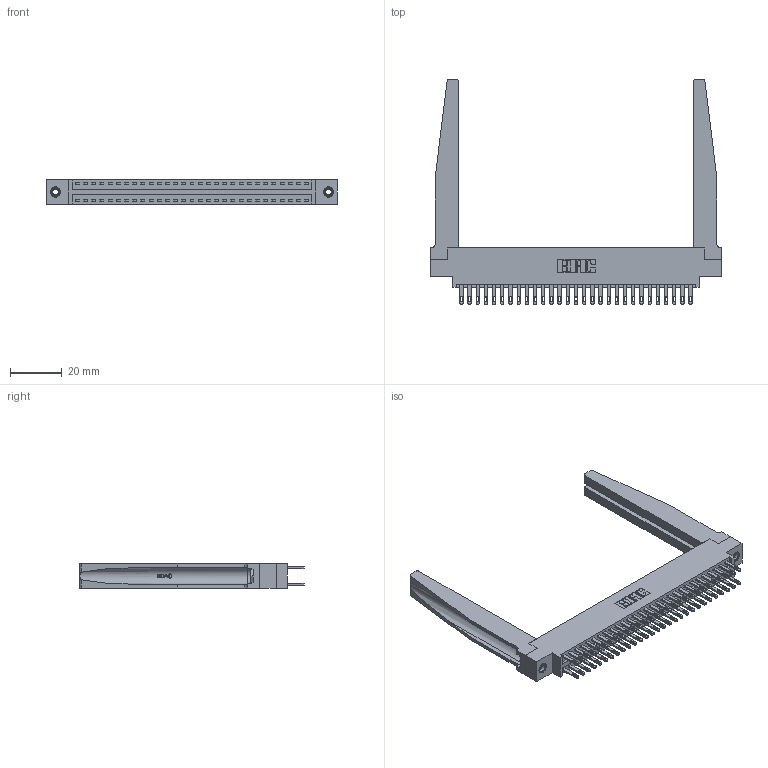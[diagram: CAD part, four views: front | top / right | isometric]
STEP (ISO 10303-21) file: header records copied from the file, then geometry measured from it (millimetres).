
FILE_DESCRIPTION (( 'STEP AP203' ), '1' );
FILE_NAME ('346-058-500-878.STEP', '2022-05-21T07:29:34', ( '' ), ( '' ), 'SwSTEP 2.0', 'SolidWorks 2020', '' );
FILE_SCHEMA (( 'CONFIG_CONTROL_DESIGN' ));
Length unit declared in the file: inch
Products named in the file (5): 346 Part_0.170 Offset - 0.156 Dia-TH; 346-058-500-878; 345-292-001_345-293-100; 345-250-001_345-250-001-102; 346-220-078_345-220-078
Assembly tree (63 placements, depth 2):
  346-058-500-878
    346 Part_0.170 Offset - 0.156 Dia-TH
    345-292-001_345-293-100  x58
    346-220-078_345-220-078  x2
    345-250-001_345-250-001-102  x2
Bounding box: 112.65 x 87.12 x 9.4 mm (x, y, z)
Volume: 17797.1 mm3; surface area: 22121 mm2
Topology: 63 solids, 63 shells, 3158 faces, 9511 edges, 6330 vertices
Faces by surface type: plane 1918, cylinder 1188, bspline 36, cone 12, torus 4
Entity records: 25902 total; most frequent: CARTESIAN_POINT 5229, ORIENTED_EDGE 4050, DIRECTION 3647, EDGE_CURVE 2025, VECTOR 1679, LINE 1679, VERTEX_POINT 1344, AXIS2_PLACEMENT_3D 984
